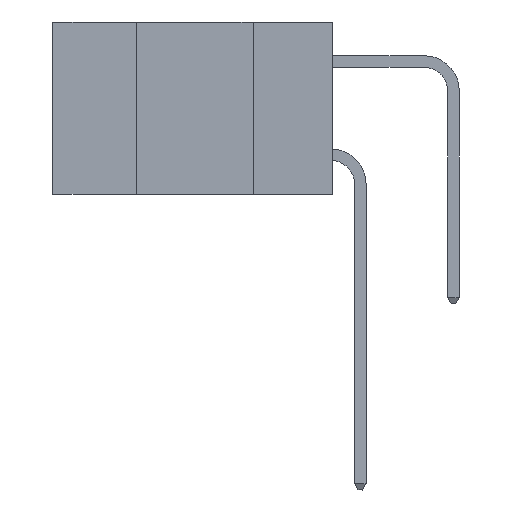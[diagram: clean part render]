
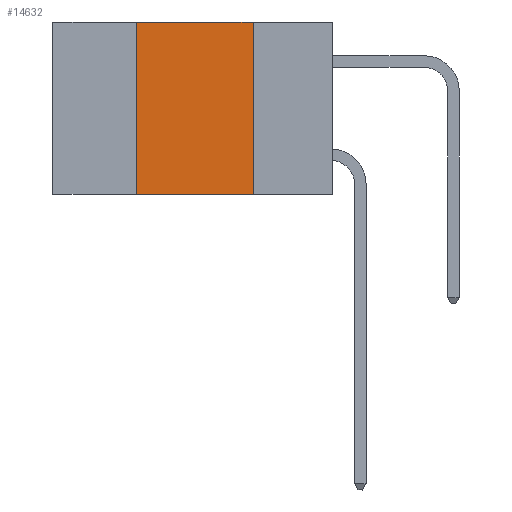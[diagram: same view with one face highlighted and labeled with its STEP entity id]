
A CAD part, left-side view. The second image highlights one B-rep face of the part: STEP entity #14632.
In plain terms, the highlighted planar face has unit normal (-1, 0, 0).
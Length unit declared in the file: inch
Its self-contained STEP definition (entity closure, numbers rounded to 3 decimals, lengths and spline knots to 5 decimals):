
#1600 = LINE ( 'NONE', #26791, #21193 ) ;
#1602 = VERTEX_POINT ( 'NONE', #3685 ) ;
#2117 = EDGE_CURVE ( 'NONE', #14602, #1602, #21254, .T. ) ;
#2388 = DIRECTION ( 'NONE',  ( 0., -1., 0. ) ) ;
#3212 = ORIENTED_EDGE ( 'NONE', *, *, #9211, .T. ) ;
#3685 = CARTESIAN_POINT ( 'NONE',  ( 0., 0.42, 0. ) ) ;
#4007 = VERTEX_POINT ( 'NONE', #17836 ) ;
#4554 = DIRECTION ( 'NONE',  ( 0., -1., 0. ) ) ;
#6509 = CARTESIAN_POINT ( 'NONE',  ( 0., 0.42, -0.37 ) ) ;
#7134 = ORIENTED_EDGE ( 'NONE', *, *, #2117, .F. ) ;
#8443 = CARTESIAN_POINT ( 'NONE',  ( 0., 0.17, 0. ) ) ;
#9211 = EDGE_CURVE ( 'NONE', #14602, #20426, #18312, .T. ) ;
#10347 = EDGE_CURVE ( 'NONE', #1602, #4007, #1600, .T. ) ;
#14602 = VERTEX_POINT ( 'NONE', #6509 ) ;
#14632 = ADVANCED_FACE ( 'NONE', ( #23696 ), #16759, .F. ) ;
#15217 = CARTESIAN_POINT ( 'NONE',  ( 0., 0.6, -0.37 ) ) ;
#16536 = CARTESIAN_POINT ( 'NONE',  ( 0., 0.42, 0. ) ) ;
#16546 = AXIS2_PLACEMENT_3D ( 'NONE', #24491, #21606, #19119 ) ;
#16759 = PLANE ( 'NONE',  #16546 ) ;
#17524 = VECTOR ( 'NONE', #2388, 39.37008 ) ;
#17836 = CARTESIAN_POINT ( 'NONE',  ( 0., 0.17, 0. ) ) ;
#18166 = DIRECTION ( 'NONE',  ( 0., 0., -1. ) ) ;
#18312 = LINE ( 'NONE', #15217, #17524 ) ;
#19119 = DIRECTION ( 'NONE',  ( 0., 0., -1. ) ) ;
#19140 = ORIENTED_EDGE ( 'NONE', *, *, #10347, .F. ) ;
#19243 = VECTOR ( 'NONE', #24019, 39.37008 ) ;
#20426 = VERTEX_POINT ( 'NONE', #24483 ) ;
#20706 = VECTOR ( 'NONE', #18166, 39.37008 ) ;
#21193 = VECTOR ( 'NONE', #4554, 39.37008 ) ;
#21254 = LINE ( 'NONE', #16536, #19243 ) ;
#21606 = DIRECTION ( 'NONE',  ( 1., 0., 0. ) ) ;
#23123 = LINE ( 'NONE', #8443, #20706 ) ;
#23696 = FACE_OUTER_BOUND ( 'NONE', #27485, .T. ) ;
#24019 = DIRECTION ( 'NONE',  ( 0., 0., 1. ) ) ;
#24483 = CARTESIAN_POINT ( 'NONE',  ( 0., 0.17, -0.37 ) ) ;
#24491 = CARTESIAN_POINT ( 'NONE',  ( 0., 0.6, 0. ) ) ;
#26791 = CARTESIAN_POINT ( 'NONE',  ( 0., 0.6, 0. ) ) ;
#27475 = ORIENTED_EDGE ( 'NONE', *, *, #31752, .F. ) ;
#27485 = EDGE_LOOP ( 'NONE', ( #27475, #19140, #7134, #3212 ) ) ;
#31752 = EDGE_CURVE ( 'NONE', #4007, #20426, #23123, .T. ) ;
